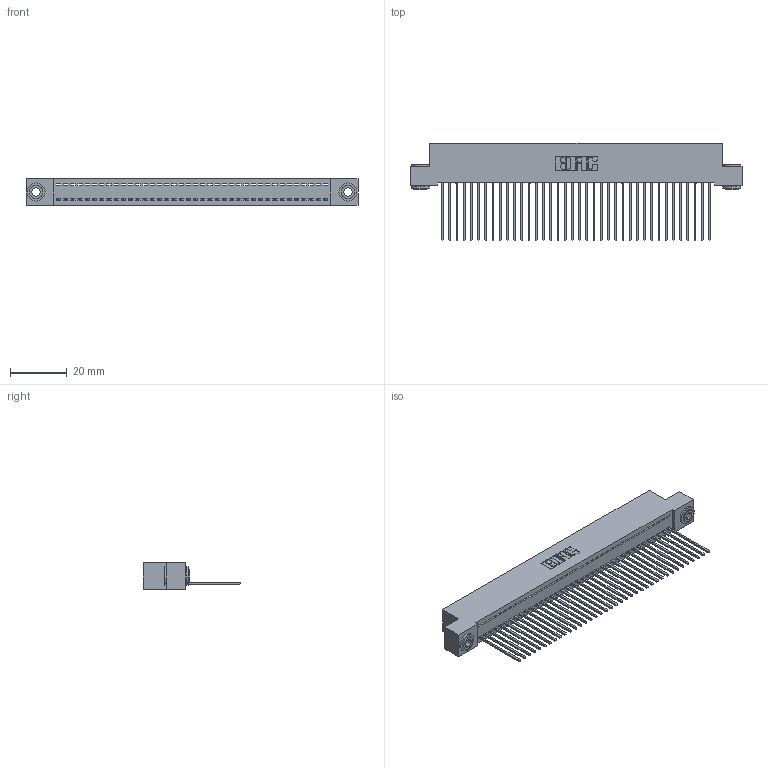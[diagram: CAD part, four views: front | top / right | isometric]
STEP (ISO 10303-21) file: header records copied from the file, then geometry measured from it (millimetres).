
FILE_DESCRIPTION (( 'STEP AP203' ), '1' );
FILE_NAME ('342-038-541-103.STEP', '2018-08-11T22:18:20', ( '' ), ( '' ), 'SwSTEP 2.0', 'SolidWorks 2016', '' );
FILE_SCHEMA (( 'CONFIG_CONTROL_DESIGN' ));
Length unit declared in the file: inch
Products named in the file (4): 342 Part_.156 TH; 345-292-001_345-293-141; 342-250-002_345-250-002-102; 342-038-541-103
Assembly tree (41 placements, depth 2):
  342-038-541-103
    342 Part_.156 TH
    345-292-001_345-293-141  x38
    342-250-002_345-250-002-102  x2
Bounding box: 116.84 x 34.3 x 9.4 mm (x, y, z)
Volume: 10378 mm3; surface area: 16104.2 mm2
Topology: 41 solids, 41 shells, 2352 faces, 7063 edges, 4654 vertices
Faces by surface type: plane 1672, cylinder 672, cone 8
Entity records: 24284 total; most frequent: CARTESIAN_POINT 4167, ORIENTED_EDGE 4134, DIRECTION 3557, EDGE_CURVE 2067, VECTOR 1915, LINE 1915, VERTEX_POINT 1374, AXIS2_PLACEMENT_3D 821
